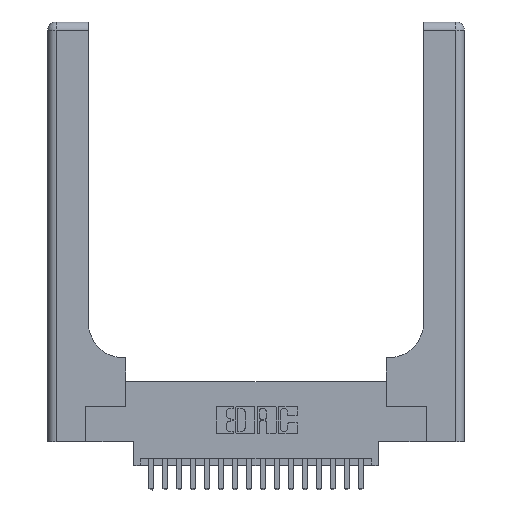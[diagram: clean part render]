
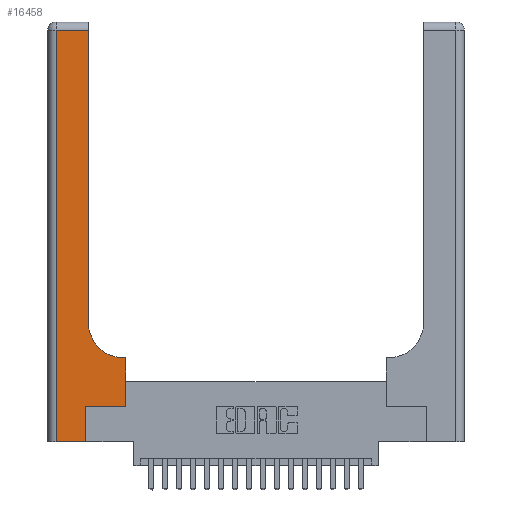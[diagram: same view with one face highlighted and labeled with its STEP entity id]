
A CAD part, top view. The second image highlights one B-rep face of the part: STEP entity #16458.
In plain terms, the highlighted planar face has unit normal (0, 0, 1).
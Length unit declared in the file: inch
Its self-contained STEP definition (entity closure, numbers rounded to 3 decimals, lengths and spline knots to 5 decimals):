
#403 = ORIENTED_EDGE ( 'NONE', *, *, #3658, .T. ) ;
#545 = EDGE_CURVE ( 'NONE', #959, #10068, #17820, .T. ) ;
#711 = CARTESIAN_POINT ( 'NONE',  ( 0.5415, 0.6, 0.37 ) ) ;
#846 = EDGE_CURVE ( 'NONE', #19622, #959, #17020, .T. ) ;
#929 = EDGE_CURVE ( 'NONE', #19966, #21401, #18067, .T. ) ;
#959 = VERTEX_POINT ( 'NONE', #4754 ) ;
#2160 = CARTESIAN_POINT ( 'NONE',  ( 0.2915, 0.85, 0.37 ) ) ;
#2356 = ORIENTED_EDGE ( 'NONE', *, *, #18941, .T. ) ;
#3167 = DIRECTION ( 'NONE',  ( 0., 1., 0. ) ) ;
#3172 = CARTESIAN_POINT ( 'NONE',  ( 0.2915, 2.94, 0.37 ) ) ;
#3279 = LINE ( 'NONE', #9875, #11815 ) ;
#3640 = CARTESIAN_POINT ( 'NONE',  ( 0., 3., 0.37 ) ) ;
#3658 = EDGE_CURVE ( 'NONE', #21401, #5206, #10351, .T. ) ;
#4754 = CARTESIAN_POINT ( 'NONE',  ( 0.06, 2.94, 0.37 ) ) ;
#5205 = VECTOR ( 'NONE', #7065, 39.37008 ) ;
#5206 = VERTEX_POINT ( 'NONE', #21062 ) ;
#5282 = ORIENTED_EDGE ( 'NONE', *, *, #929, .T. ) ;
#5405 = CARTESIAN_POINT ( 'NONE',  ( 0.06, 3., 0.37 ) ) ;
#5975 = VECTOR ( 'NONE', #6128, 39.37008 ) ;
#6128 = DIRECTION ( 'NONE',  ( 1., 0., 0. ) ) ;
#6229 = ORIENTED_EDGE ( 'NONE', *, *, #17492, .T. ) ;
#6638 = EDGE_CURVE ( 'NONE', #10068, #19966, #3279, .T. ) ;
#7065 = DIRECTION ( 'NONE',  ( 0., 1., 0. ) ) ;
#7181 = AXIS2_PLACEMENT_3D ( 'NONE', #3640, #18449, #8479 ) ;
#7229 = ORIENTED_EDGE ( 'NONE', *, *, #6638, .T. ) ;
#7568 = DIRECTION ( 'NONE',  ( 0., 0., -1. ) ) ;
#7682 = VECTOR ( 'NONE', #3167, 39.37008 ) ;
#8479 = DIRECTION ( 'NONE',  ( -1., 0., 0. ) ) ;
#8642 = LINE ( 'NONE', #14671, #11265 ) ;
#9622 = DIRECTION ( 'NONE',  ( -1., 0., 0. ) ) ;
#9875 = CARTESIAN_POINT ( 'NONE',  ( 0., 0., 0.37 ) ) ;
#10068 = VERTEX_POINT ( 'NONE', #20436 ) ;
#10351 = LINE ( 'NONE', #14362, #5975 ) ;
#10426 = ORIENTED_EDGE ( 'NONE', *, *, #21092, .T. ) ;
#10979 = CARTESIAN_POINT ( 'NONE',  ( 0.269, 0., 0.37 ) ) ;
#11265 = VECTOR ( 'NONE', #17937, 39.37008 ) ;
#11493 = VERTEX_POINT ( 'NONE', #21309 ) ;
#11519 = ORIENTED_EDGE ( 'NONE', *, *, #545, .T. ) ;
#11612 = VECTOR ( 'NONE', #16691, 39.37008 ) ;
#11815 = VECTOR ( 'NONE', #14098, 39.37008 ) ;
#12091 = VECTOR ( 'NONE', #9622, 39.37008 ) ;
#12095 = VECTOR ( 'NONE', #19359, 39.37008 ) ;
#12186 = CIRCLE ( 'NONE', #20412, 0.25 ) ;
#12555 = CARTESIAN_POINT ( 'NONE',  ( 0.5415, 0.85, 0.37 ) ) ;
#13954 = ORIENTED_EDGE ( 'NONE', *, *, #846, .T. ) ;
#14098 = DIRECTION ( 'NONE',  ( 1., 0., 0. ) ) ;
#14355 = CARTESIAN_POINT ( 'NONE',  ( 0.269, 0.25, 0.37 ) ) ;
#14362 = CARTESIAN_POINT ( 'NONE',  ( 0.269, 0.25, 0.37 ) ) ;
#14366 = DIRECTION ( 'NONE',  ( 1., 0., 0. ) ) ;
#14671 = CARTESIAN_POINT ( 'NONE',  ( 0.5585, 0.25, 0.37 ) ) ;
#14765 = VERTEX_POINT ( 'NONE', #2160 ) ;
#14952 = EDGE_LOOP ( 'NONE', ( #19068, #13954, #11519, #7229, #5282, #403, #10426, #2356, #6229 ) ) ;
#16111 = CARTESIAN_POINT ( 'NONE',  ( 0., 2.94, 0.37 ) ) ;
#16398 = CARTESIAN_POINT ( 'NONE',  ( 0.269, 0., 0.37 ) ) ;
#16458 = ADVANCED_FACE ( 'NONE', ( #16621 ), #19975, .F. ) ;
#16621 = FACE_OUTER_BOUND ( 'NONE', #14952, .T. ) ;
#16691 = DIRECTION ( 'NONE',  ( 0., -1., 0. ) ) ;
#16825 = EDGE_CURVE ( 'NONE', #14765, #19622, #16852, .T. ) ;
#16852 = LINE ( 'NONE', #18172, #5205 ) ;
#17020 = LINE ( 'NONE', #16111, #12095 ) ;
#17492 = EDGE_CURVE ( 'NONE', #20856, #14765, #12186, .T. ) ;
#17820 = LINE ( 'NONE', #5405, #11612 ) ;
#17912 = CARTESIAN_POINT ( 'NONE',  ( 0.2915, 0.6, 0.37 ) ) ;
#17937 = DIRECTION ( 'NONE',  ( 0., 1., 0. ) ) ;
#18067 = LINE ( 'NONE', #16398, #7682 ) ;
#18172 = CARTESIAN_POINT ( 'NONE',  ( 0.2915, 3., 0.37 ) ) ;
#18449 = DIRECTION ( 'NONE',  ( 0., 0., -1. ) ) ;
#18941 = EDGE_CURVE ( 'NONE', #11493, #20856, #19891, .T. ) ;
#19068 = ORIENTED_EDGE ( 'NONE', *, *, #16825, .T. ) ;
#19359 = DIRECTION ( 'NONE',  ( -1., 0., 0. ) ) ;
#19622 = VERTEX_POINT ( 'NONE', #3172 ) ;
#19891 = LINE ( 'NONE', #17912, #12091 ) ;
#19966 = VERTEX_POINT ( 'NONE', #10979 ) ;
#19975 = PLANE ( 'NONE',  #7181 ) ;
#20412 = AXIS2_PLACEMENT_3D ( 'NONE', #12555, #7568, #14366 ) ;
#20436 = CARTESIAN_POINT ( 'NONE',  ( 0.06, 0., 0.37 ) ) ;
#20856 = VERTEX_POINT ( 'NONE', #711 ) ;
#21062 = CARTESIAN_POINT ( 'NONE',  ( 0.5585, 0.25, 0.37 ) ) ;
#21092 = EDGE_CURVE ( 'NONE', #5206, #11493, #8642, .T. ) ;
#21309 = CARTESIAN_POINT ( 'NONE',  ( 0.5585, 0.6, 0.37 ) ) ;
#21401 = VERTEX_POINT ( 'NONE', #14355 ) ;
